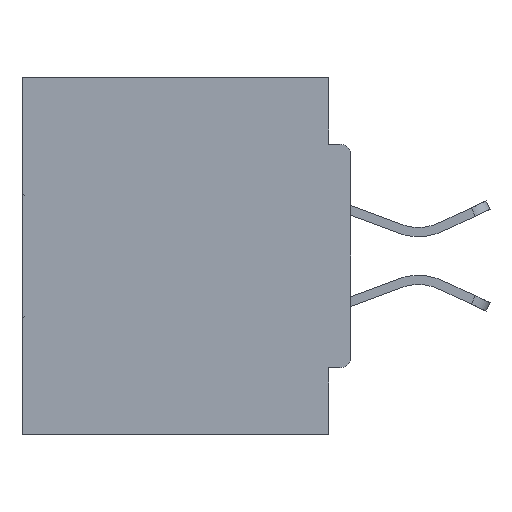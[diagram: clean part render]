
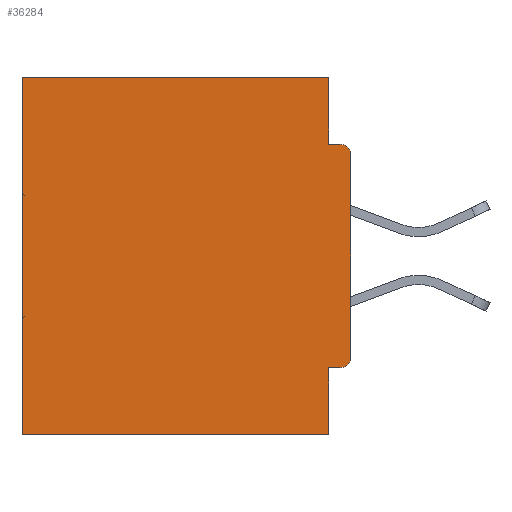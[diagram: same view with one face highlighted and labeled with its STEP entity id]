
A CAD part, left-side view. The second image highlights one B-rep face of the part: STEP entity #36284.
In plain terms, the highlighted planar face has unit normal (-1, 0, 0).
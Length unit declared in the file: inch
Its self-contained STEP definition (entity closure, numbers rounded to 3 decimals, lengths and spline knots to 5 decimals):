
#283 = VERTEX_POINT ( 'NONE', #28433 ) ;
#2593 = LINE ( 'NONE', #18191, #37307 ) ;
#2759 = EDGE_CURVE ( 'NONE', #15100, #8333, #37962, .T. ) ;
#2764 = CARTESIAN_POINT ( 'NONE',  ( 0.298, 0.46, 0. ) ) ;
#3014 = LINE ( 'NONE', #30586, #4090 ) ;
#3529 = CIRCLE ( 'NONE', #4343, 0.015 ) ;
#3949 = CARTESIAN_POINT ( 'NONE',  ( 0.298, 0., -0.0935 ) ) ;
#3971 = CARTESIAN_POINT ( 'NONE',  ( 0.298, 0.015, -0.0935 ) ) ;
#4090 = VECTOR ( 'NONE', #13981, 39.37008 ) ;
#4343 = AXIS2_PLACEMENT_3D ( 'NONE', #34653, #7627, #34950 ) ;
#4927 = DIRECTION ( 'NONE',  ( 0., 1., 0. ) ) ;
#5088 = DIRECTION ( 'NONE',  ( 0., 0., -1. ) ) ;
#5451 = VERTEX_POINT ( 'NONE', #3971 ) ;
#5818 = ORIENTED_EDGE ( 'NONE', *, *, #39981, .F. ) ;
#6891 = ORIENTED_EDGE ( 'NONE', *, *, #40974, .F. ) ;
#7490 = ORIENTED_EDGE ( 'NONE', *, *, #17084, .F. ) ;
#7627 = DIRECTION ( 'NONE',  ( -1., 0., 0. ) ) ;
#8333 = VERTEX_POINT ( 'NONE', #42681 ) ;
#8522 = LINE ( 'NONE', #2764, #34318 ) ;
#8678 = LINE ( 'NONE', #22129, #40798 ) ;
#10023 = AXIS2_PLACEMENT_3D ( 'NONE', #38828, #18734, #42198 ) ;
#10135 = FACE_OUTER_BOUND ( 'NONE', #39141, .T. ) ;
#11232 = EDGE_CURVE ( 'NONE', #15100, #283, #3014, .T. ) ;
#11601 = EDGE_CURVE ( 'NONE', #20316, #5451, #3529, .T. ) ;
#12107 = CARTESIAN_POINT ( 'NONE',  ( 0.298, 0.031, -0.5 ) ) ;
#12143 = AXIS2_PLACEMENT_3D ( 'NONE', #42870, #29678, #12875 ) ;
#12875 = DIRECTION ( 'NONE',  ( 0., 0., -1. ) ) ;
#13347 = ORIENTED_EDGE ( 'NONE', *, *, #42691, .T. ) ;
#13981 = DIRECTION ( 'NONE',  ( 0., 1., 0. ) ) ;
#15093 = LINE ( 'NONE', #25659, #16679 ) ;
#15100 = VERTEX_POINT ( 'NONE', #37384 ) ;
#15964 = ORIENTED_EDGE ( 'NONE', *, *, #17998, .T. ) ;
#16202 = VECTOR ( 'NONE', #39753, 39.37008 ) ;
#16679 = VECTOR ( 'NONE', #5088, 39.37008 ) ;
#17084 = EDGE_CURVE ( 'NONE', #283, #40645, #17991, .T. ) ;
#17991 = LINE ( 'NONE', #40936, #31096 ) ;
#17998 = EDGE_CURVE ( 'NONE', #24512, #41882, #2593, .T. ) ;
#18007 = VERTEX_POINT ( 'NONE', #24799 ) ;
#18191 = CARTESIAN_POINT ( 'NONE',  ( 0.298, 0., 0. ) ) ;
#18532 = CARTESIAN_POINT ( 'NONE',  ( 0.298, 0.031, 0. ) ) ;
#18734 = DIRECTION ( 'NONE',  ( 1., 0., 0. ) ) ;
#20316 = VERTEX_POINT ( 'NONE', #23075 ) ;
#22129 = CARTESIAN_POINT ( 'NONE',  ( 0.298, 0., -0.5 ) ) ;
#22430 = PLANE ( 'NONE',  #10023 ) ;
#23072 = VECTOR ( 'NONE', #33905, 39.37008 ) ;
#23075 = CARTESIAN_POINT ( 'NONE',  ( 0.298, 0., -0.1085 ) ) ;
#23682 = ORIENTED_EDGE ( 'NONE', *, *, #2759, .T. ) ;
#24512 = VERTEX_POINT ( 'NONE', #18532 ) ;
#24799 = CARTESIAN_POINT ( 'NONE',  ( 0.298, 0.031, -0.0935 ) ) ;
#25659 = CARTESIAN_POINT ( 'NONE',  ( 0.298, 0., 0. ) ) ;
#26084 = CARTESIAN_POINT ( 'NONE',  ( 0.298, 0.46, 0. ) ) ;
#27264 = LINE ( 'NONE', #12107, #16202 ) ;
#28166 = CARTESIAN_POINT ( 'NONE',  ( 0.298, 0.031, -0.5 ) ) ;
#28433 = CARTESIAN_POINT ( 'NONE',  ( 0.298, 0.031, -0.4065 ) ) ;
#29344 = EDGE_CURVE ( 'NONE', #20316, #8333, #15093, .T. ) ;
#29678 = DIRECTION ( 'NONE',  ( -1., 0., 0. ) ) ;
#30191 = VERTEX_POINT ( 'NONE', #34902 ) ;
#30586 = CARTESIAN_POINT ( 'NONE',  ( 0.298, 0., -0.4065 ) ) ;
#30930 = ORIENTED_EDGE ( 'NONE', *, *, #40113, .F. ) ;
#31096 = VECTOR ( 'NONE', #31105, 39.37008 ) ;
#31105 = DIRECTION ( 'NONE',  ( 0., 0., -1. ) ) ;
#31961 = LINE ( 'NONE', #3949, #23072 ) ;
#33451 = DIRECTION ( 'NONE',  ( 0., 0., -1. ) ) ;
#33905 = DIRECTION ( 'NONE',  ( 0., -1., 0. ) ) ;
#34318 = VECTOR ( 'NONE', #33451, 39.37008 ) ;
#34653 = CARTESIAN_POINT ( 'NONE',  ( 0.298, 0.015, -0.1085 ) ) ;
#34902 = CARTESIAN_POINT ( 'NONE',  ( 0.298, 0.46, -0.5 ) ) ;
#34950 = DIRECTION ( 'NONE',  ( 0., 0., -1. ) ) ;
#36284 = ADVANCED_FACE ( 'NONE', ( #10135 ), #22430, .F. ) ;
#37307 = VECTOR ( 'NONE', #4927, 39.37008 ) ;
#37384 = CARTESIAN_POINT ( 'NONE',  ( 0.298, 0.015, -0.4065 ) ) ;
#37962 = CIRCLE ( 'NONE', #12143, 0.015 ) ;
#38828 = CARTESIAN_POINT ( 'NONE',  ( 0.298, 0., 0. ) ) ;
#39126 = ORIENTED_EDGE ( 'NONE', *, *, #29344, .F. ) ;
#39141 = EDGE_LOOP ( 'NONE', ( #40547, #30930, #5818, #15964, #13347, #6891, #7490, #43295, #23682, #39126 ) ) ;
#39753 = DIRECTION ( 'NONE',  ( 0., 0., -1. ) ) ;
#39981 = EDGE_CURVE ( 'NONE', #24512, #18007, #27264, .T. ) ;
#40113 = EDGE_CURVE ( 'NONE', #18007, #5451, #31961, .T. ) ;
#40547 = ORIENTED_EDGE ( 'NONE', *, *, #11601, .T. ) ;
#40645 = VERTEX_POINT ( 'NONE', #28166 ) ;
#40798 = VECTOR ( 'NONE', #42992, 39.37008 ) ;
#40936 = CARTESIAN_POINT ( 'NONE',  ( 0.298, 0.031, -0.5 ) ) ;
#40974 = EDGE_CURVE ( 'NONE', #40645, #30191, #8678, .T. ) ;
#41882 = VERTEX_POINT ( 'NONE', #26084 ) ;
#42198 = DIRECTION ( 'NONE',  ( 0., 0., -1. ) ) ;
#42681 = CARTESIAN_POINT ( 'NONE',  ( 0.298, 0., -0.3915 ) ) ;
#42691 = EDGE_CURVE ( 'NONE', #41882, #30191, #8522, .T. ) ;
#42870 = CARTESIAN_POINT ( 'NONE',  ( 0.298, 0.015, -0.3915 ) ) ;
#42992 = DIRECTION ( 'NONE',  ( 0., 1., 0. ) ) ;
#43295 = ORIENTED_EDGE ( 'NONE', *, *, #11232, .F. ) ;
